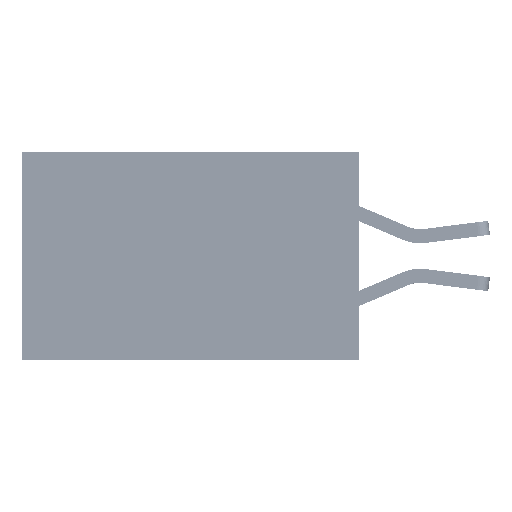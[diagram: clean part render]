
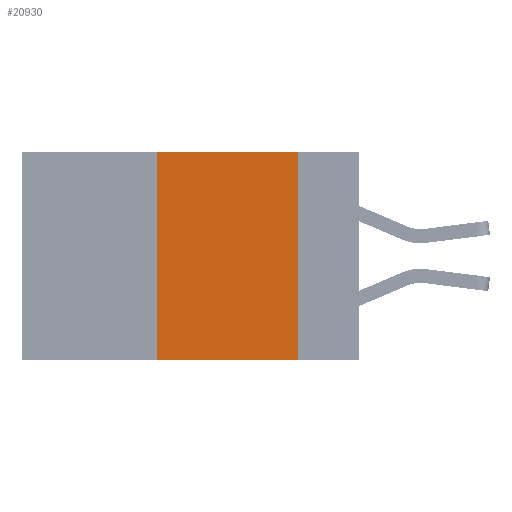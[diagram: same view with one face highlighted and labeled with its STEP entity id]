
A CAD part, left-side view. The second image highlights one B-rep face of the part: STEP entity #20930.
In plain terms, the highlighted planar face has unit normal (-1, 0, 0).
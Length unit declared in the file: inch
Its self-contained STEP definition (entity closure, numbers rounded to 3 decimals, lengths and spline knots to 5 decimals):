
#669 = ORIENTED_EDGE ( 'NONE', *, *, #7339, .T. ) ;
#1856 = DIRECTION ( 'NONE',  ( 0., 0., -1. ) ) ;
#2385 = CARTESIAN_POINT ( 'NONE',  ( 0., 0.6, -0.37 ) ) ;
#5486 = PLANE ( 'NONE',  #14828 ) ;
#6297 = CARTESIAN_POINT ( 'NONE',  ( 0., 0.11, 0. ) ) ;
#7339 = EDGE_CURVE ( 'NONE', #35410, #21697, #38238, .T. ) ;
#8243 = CARTESIAN_POINT ( 'NONE',  ( 0., 0.36, -0.37 ) ) ;
#10979 = ORIENTED_EDGE ( 'NONE', *, *, #26124, .F. ) ;
#11341 = LINE ( 'NONE', #12920, #20517 ) ;
#11376 = DIRECTION ( 'NONE',  ( 0., -1., 0. ) ) ;
#12920 = CARTESIAN_POINT ( 'NONE',  ( 0., 0.36, 0. ) ) ;
#13158 = FACE_OUTER_BOUND ( 'NONE', #31918, .T. ) ;
#14828 = AXIS2_PLACEMENT_3D ( 'NONE', #20686, #35937, #1856 ) ;
#15235 = CARTESIAN_POINT ( 'NONE',  ( 0., 0.11, -0.37 ) ) ;
#16022 = ORIENTED_EDGE ( 'NONE', *, *, #32426, .F. ) ;
#16904 = DIRECTION ( 'NONE',  ( 0., -1., 0. ) ) ;
#18846 = VECTOR ( 'NONE', #31241, 39.37008 ) ;
#18961 = CARTESIAN_POINT ( 'NONE',  ( 0., 0.36, 0. ) ) ;
#20466 = VERTEX_POINT ( 'NONE', #18961 ) ;
#20517 = VECTOR ( 'NONE', #25385, 39.37008 ) ;
#20686 = CARTESIAN_POINT ( 'NONE',  ( 0., 0.6, 0. ) ) ;
#20930 = ADVANCED_FACE ( 'NONE', ( #13158 ), #5486, .F. ) ;
#21697 = VERTEX_POINT ( 'NONE', #15235 ) ;
#22307 = EDGE_CURVE ( 'NONE', #37397, #21697, #27122, .T. ) ;
#22829 = LINE ( 'NONE', #25720, #32484 ) ;
#25385 = DIRECTION ( 'NONE',  ( 0., 0., 1. ) ) ;
#25720 = CARTESIAN_POINT ( 'NONE',  ( 0., 0.6, 0. ) ) ;
#26124 = EDGE_CURVE ( 'NONE', #35410, #20466, #11341, .T. ) ;
#26187 = VECTOR ( 'NONE', #11376, 39.37008 ) ;
#27122 = LINE ( 'NONE', #6297, #18846 ) ;
#27973 = ORIENTED_EDGE ( 'NONE', *, *, #22307, .F. ) ;
#31241 = DIRECTION ( 'NONE',  ( 0., 0., -1. ) ) ;
#31918 = EDGE_LOOP ( 'NONE', ( #27973, #16022, #10979, #669 ) ) ;
#32426 = EDGE_CURVE ( 'NONE', #20466, #37397, #22829, .T. ) ;
#32484 = VECTOR ( 'NONE', #16904, 39.37008 ) ;
#35410 = VERTEX_POINT ( 'NONE', #8243 ) ;
#35937 = DIRECTION ( 'NONE',  ( 1., 0., 0. ) ) ;
#35979 = CARTESIAN_POINT ( 'NONE',  ( 0., 0.11, 0. ) ) ;
#37397 = VERTEX_POINT ( 'NONE', #35979 ) ;
#38238 = LINE ( 'NONE', #2385, #26187 ) ;
